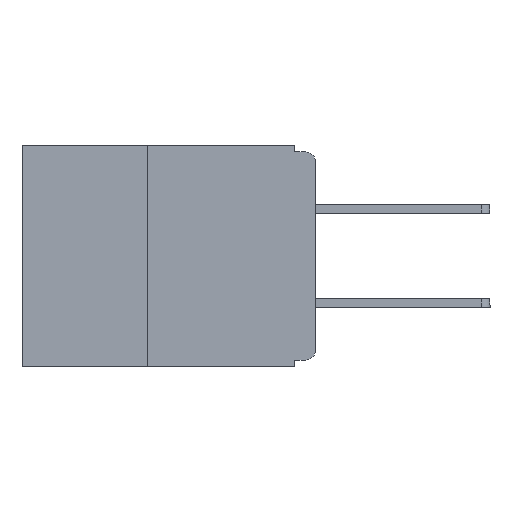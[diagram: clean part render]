
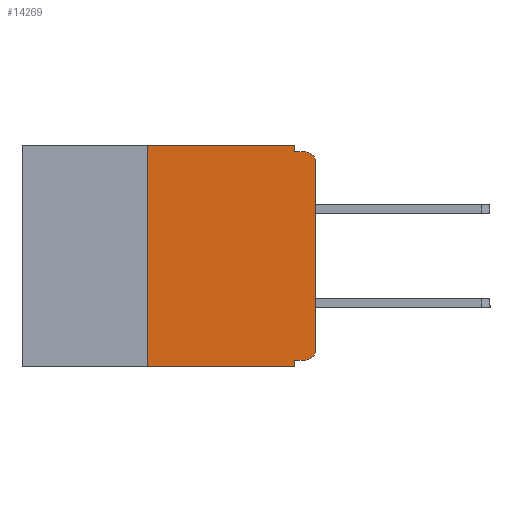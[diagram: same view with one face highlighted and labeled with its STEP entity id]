
A CAD part, left-side view. The second image highlights one B-rep face of the part: STEP entity #14269.
In plain terms, the highlighted planar face has unit normal (-1, 0, 0).
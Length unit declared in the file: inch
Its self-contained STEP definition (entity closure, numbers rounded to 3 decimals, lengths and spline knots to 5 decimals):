
#482 = CARTESIAN_POINT ( 'NONE',  ( 0., 0.015, -0.01 ) ) ;
#498 = CARTESIAN_POINT ( 'NONE',  ( 0., 0.015, -0.32 ) ) ;
#1066 = CARTESIAN_POINT ( 'NONE',  ( 0., 0.031, 0. ) ) ;
#1227 = DIRECTION ( 'NONE',  ( 0., -1., 0. ) ) ;
#1258 = CARTESIAN_POINT ( 'NONE',  ( 0., 0.25, -0.33 ) ) ;
#1344 = DIRECTION ( 'NONE',  ( 0., 0., -1. ) ) ;
#1402 = CARTESIAN_POINT ( 'NONE',  ( 0., 0.437, -0.33 ) ) ;
#1632 = ORIENTED_EDGE ( 'NONE', *, *, #3059, .F. ) ;
#2160 = CARTESIAN_POINT ( 'NONE',  ( 0., 0.015, -0.305 ) ) ;
#2189 = LINE ( 'NONE', #11634, #6043 ) ;
#2309 = ORIENTED_EDGE ( 'NONE', *, *, #4299, .F. ) ;
#2417 = VECTOR ( 'NONE', #1227, 39.37008 ) ;
#2528 = DIRECTION ( 'NONE',  ( 0., 0., 1. ) ) ;
#3059 = EDGE_CURVE ( 'NONE', #3758, #7358, #14869, .T. ) ;
#3244 = ORIENTED_EDGE ( 'NONE', *, *, #4818, .T. ) ;
#3284 = AXIS2_PLACEMENT_3D ( 'NONE', #6492, #9071, #1344 ) ;
#3293 = CARTESIAN_POINT ( 'NONE',  ( 0., 0.25, -0.33 ) ) ;
#3353 = VERTEX_POINT ( 'NONE', #482 ) ;
#3426 = DIRECTION ( 'NONE',  ( 0., 0., -1. ) ) ;
#3540 = CARTESIAN_POINT ( 'NONE',  ( 0., 0.031, -0.01 ) ) ;
#3758 = VERTEX_POINT ( 'NONE', #12590 ) ;
#3784 = AXIS2_PLACEMENT_3D ( 'NONE', #2160, #11159, #3426 ) ;
#3911 = DIRECTION ( 'NONE',  ( 0., -1., 0. ) ) ;
#4016 = VERTEX_POINT ( 'NONE', #10115 ) ;
#4299 = EDGE_CURVE ( 'NONE', #11434, #3758, #10117, .T. ) ;
#4818 = EDGE_CURVE ( 'NONE', #8712, #7358, #5874, .T. ) ;
#5168 = PLANE ( 'NONE',  #3284 ) ;
#5352 = LINE ( 'NONE', #1066, #12152 ) ;
#5494 = DIRECTION ( 'NONE',  ( -1., 0., 0. ) ) ;
#5874 = LINE ( 'NONE', #1402, #2417 ) ;
#6043 = VECTOR ( 'NONE', #3911, 39.37008 ) ;
#6422 = VERTEX_POINT ( 'NONE', #16160 ) ;
#6492 = CARTESIAN_POINT ( 'NONE',  ( 0., 0.437, 0. ) ) ;
#6754 = ORIENTED_EDGE ( 'NONE', *, *, #8127, .T. ) ;
#6812 = CARTESIAN_POINT ( 'NONE',  ( 0., 0., -0.32 ) ) ;
#6886 = DIRECTION ( 'NONE',  ( 0., 1., 0. ) ) ;
#7358 = VERTEX_POINT ( 'NONE', #11998 ) ;
#7744 = VECTOR ( 'NONE', #7767, 39.37008 ) ;
#7767 = DIRECTION ( 'NONE',  ( 0., 0., -1. ) ) ;
#7808 = CARTESIAN_POINT ( 'NONE',  ( 0., 0.031, -0.33 ) ) ;
#7998 = DIRECTION ( 'NONE',  ( 0., -1., 0. ) ) ;
#8127 = EDGE_CURVE ( 'NONE', #11434, #4016, #14886, .T. ) ;
#8310 = EDGE_CURVE ( 'NONE', #8712, #8960, #12753, .T. ) ;
#8352 = EDGE_CURVE ( 'NONE', #4016, #6422, #11961, .T. ) ;
#8712 = VERTEX_POINT ( 'NONE', #3293 ) ;
#8960 = VERTEX_POINT ( 'NONE', #10255 ) ;
#9002 = VECTOR ( 'NONE', #14114, 39.37008 ) ;
#9071 = DIRECTION ( 'NONE',  ( 1., 0., 0. ) ) ;
#9099 = ORIENTED_EDGE ( 'NONE', *, *, #8352, .T. ) ;
#9414 = ORIENTED_EDGE ( 'NONE', *, *, #14891, .T. ) ;
#9488 = FACE_OUTER_BOUND ( 'NONE', #12951, .T. ) ;
#9587 = AXIS2_PLACEMENT_3D ( 'NONE', #13141, #5494, #14397 ) ;
#9708 = VECTOR ( 'NONE', #6886, 39.37008 ) ;
#10001 = VERTEX_POINT ( 'NONE', #3540 ) ;
#10075 = DIRECTION ( 'NONE',  ( 0., 0., -1. ) ) ;
#10115 = CARTESIAN_POINT ( 'NONE',  ( 0., 0., -0.305 ) ) ;
#10117 = LINE ( 'NONE', #6812, #9708 ) ;
#10255 = CARTESIAN_POINT ( 'NONE',  ( 0., 0.25, 0. ) ) ;
#10283 = CIRCLE ( 'NONE', #9587, 0.015 ) ;
#10887 = ORIENTED_EDGE ( 'NONE', *, *, #15407, .F. ) ;
#11159 = DIRECTION ( 'NONE',  ( -1., 0., 0. ) ) ;
#11344 = ORIENTED_EDGE ( 'NONE', *, *, #11696, .F. ) ;
#11434 = VERTEX_POINT ( 'NONE', #498 ) ;
#11634 = CARTESIAN_POINT ( 'NONE',  ( 0., 0., -0.01 ) ) ;
#11696 = EDGE_CURVE ( 'NONE', #16411, #10001, #5352, .T. ) ;
#11961 = LINE ( 'NONE', #12852, #9002 ) ;
#11998 = CARTESIAN_POINT ( 'NONE',  ( 0., 0.031, -0.33 ) ) ;
#12152 = VECTOR ( 'NONE', #10075, 39.37008 ) ;
#12277 = LINE ( 'NONE', #12779, #12668 ) ;
#12590 = CARTESIAN_POINT ( 'NONE',  ( 0., 0.031, -0.32 ) ) ;
#12668 = VECTOR ( 'NONE', #7998, 39.37008 ) ;
#12753 = LINE ( 'NONE', #1258, #15683 ) ;
#12779 = CARTESIAN_POINT ( 'NONE',  ( 0., 0.437, 0. ) ) ;
#12852 = CARTESIAN_POINT ( 'NONE',  ( 0., 0., 0. ) ) ;
#12951 = EDGE_LOOP ( 'NONE', ( #9099, #9414, #10887, #11344, #13071, #13883, #3244, #1632, #2309, #6754 ) ) ;
#13071 = ORIENTED_EDGE ( 'NONE', *, *, #13645, .F. ) ;
#13141 = CARTESIAN_POINT ( 'NONE',  ( 0., 0.015, -0.025 ) ) ;
#13645 = EDGE_CURVE ( 'NONE', #8960, #16411, #12277, .T. ) ;
#13883 = ORIENTED_EDGE ( 'NONE', *, *, #8310, .F. ) ;
#14114 = DIRECTION ( 'NONE',  ( 0., 0., 1. ) ) ;
#14269 = ADVANCED_FACE ( 'NONE', ( #9488 ), #5168, .F. ) ;
#14397 = DIRECTION ( 'NONE',  ( 0., 0., -1. ) ) ;
#14869 = LINE ( 'NONE', #7808, #7744 ) ;
#14886 = CIRCLE ( 'NONE', #3784, 0.015 ) ;
#14891 = EDGE_CURVE ( 'NONE', #6422, #3353, #10283, .T. ) ;
#15407 = EDGE_CURVE ( 'NONE', #10001, #3353, #2189, .T. ) ;
#15683 = VECTOR ( 'NONE', #2528, 39.37008 ) ;
#16115 = CARTESIAN_POINT ( 'NONE',  ( 0., 0.031, 0. ) ) ;
#16160 = CARTESIAN_POINT ( 'NONE',  ( 0., 0., -0.025 ) ) ;
#16411 = VERTEX_POINT ( 'NONE', #16115 ) ;
